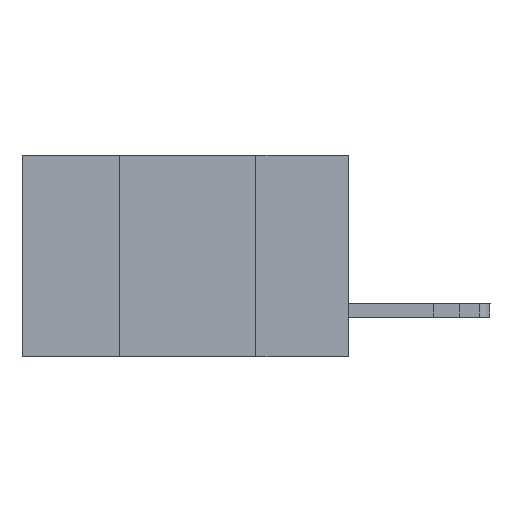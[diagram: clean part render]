
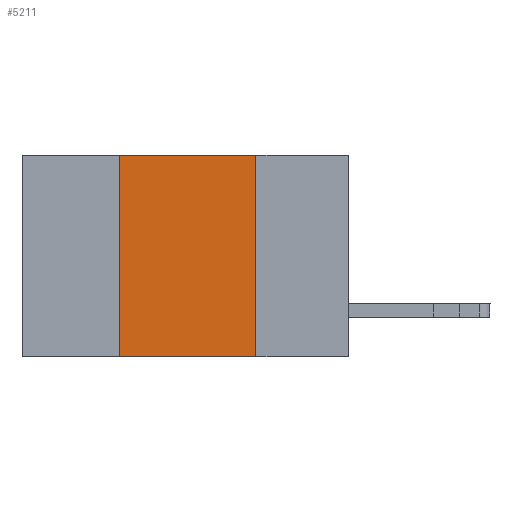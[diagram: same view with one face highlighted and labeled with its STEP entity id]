
A CAD part, left-side view. The second image highlights one B-rep face of the part: STEP entity #5211.
In plain terms, the highlighted planar face has unit normal (-1, 0, 0).
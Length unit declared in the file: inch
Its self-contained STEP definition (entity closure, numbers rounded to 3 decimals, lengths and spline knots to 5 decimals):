
#169 = CARTESIAN_POINT ( 'NONE',  ( 0., 0.42, 0. ) ) ;
#883 = VERTEX_POINT ( 'NONE', #169 ) ;
#959 = DIRECTION ( 'NONE',  ( 0., 0., -1. ) ) ;
#1187 = CARTESIAN_POINT ( 'NONE',  ( 0., 0.17, 0. ) ) ;
#1391 = ORIENTED_EDGE ( 'NONE', *, *, #11229, .T. ) ;
#1407 = VECTOR ( 'NONE', #7690, 39.37008 ) ;
#1425 = LINE ( 'NONE', #6506, #2008 ) ;
#1680 = VECTOR ( 'NONE', #5171, 39.37008 ) ;
#2008 = VECTOR ( 'NONE', #6246, 39.37008 ) ;
#2177 = LINE ( 'NONE', #8290, #11988 ) ;
#2658 = EDGE_CURVE ( 'NONE', #10454, #6711, #6026, .T. ) ;
#3256 = VERTEX_POINT ( 'NONE', #12576 ) ;
#3270 = EDGE_LOOP ( 'NONE', ( #5140, #10153, #10471, #1391 ) ) ;
#3902 = CARTESIAN_POINT ( 'NONE',  ( 0., 0.6, 0. ) ) ;
#5140 = ORIENTED_EDGE ( 'NONE', *, *, #2658, .F. ) ;
#5171 = DIRECTION ( 'NONE',  ( 0., 0., -1. ) ) ;
#5211 = ADVANCED_FACE ( 'NONE', ( #6822 ), #8847, .F. ) ;
#5742 = LINE ( 'NONE', #6834, #1407 ) ;
#6026 = LINE ( 'NONE', #1187, #1680 ) ;
#6077 = EDGE_CURVE ( 'NONE', #3256, #883, #1425, .T. ) ;
#6246 = DIRECTION ( 'NONE',  ( 0., 0., 1. ) ) ;
#6506 = CARTESIAN_POINT ( 'NONE',  ( 0., 0.42, 0. ) ) ;
#6515 = CARTESIAN_POINT ( 'NONE',  ( 0., 0.17, -0.37 ) ) ;
#6601 = CARTESIAN_POINT ( 'NONE',  ( 0., 0.17, 0. ) ) ;
#6711 = VERTEX_POINT ( 'NONE', #6515 ) ;
#6822 = FACE_OUTER_BOUND ( 'NONE', #3270, .T. ) ;
#6834 = CARTESIAN_POINT ( 'NONE',  ( 0., 0.6, -0.37 ) ) ;
#6886 = DIRECTION ( 'NONE',  ( 1., 0., 0. ) ) ;
#7690 = DIRECTION ( 'NONE',  ( 0., -1., 0. ) ) ;
#8290 = CARTESIAN_POINT ( 'NONE',  ( 0., 0.6, 0. ) ) ;
#8847 = PLANE ( 'NONE',  #9715 ) ;
#9715 = AXIS2_PLACEMENT_3D ( 'NONE', #3902, #6886, #959 ) ;
#10153 = ORIENTED_EDGE ( 'NONE', *, *, #10381, .F. ) ;
#10381 = EDGE_CURVE ( 'NONE', #883, #10454, #2177, .T. ) ;
#10454 = VERTEX_POINT ( 'NONE', #6601 ) ;
#10471 = ORIENTED_EDGE ( 'NONE', *, *, #6077, .F. ) ;
#11029 = DIRECTION ( 'NONE',  ( 0., -1., 0. ) ) ;
#11229 = EDGE_CURVE ( 'NONE', #3256, #6711, #5742, .T. ) ;
#11988 = VECTOR ( 'NONE', #11029, 39.37008 ) ;
#12576 = CARTESIAN_POINT ( 'NONE',  ( 0., 0.42, -0.37 ) ) ;
